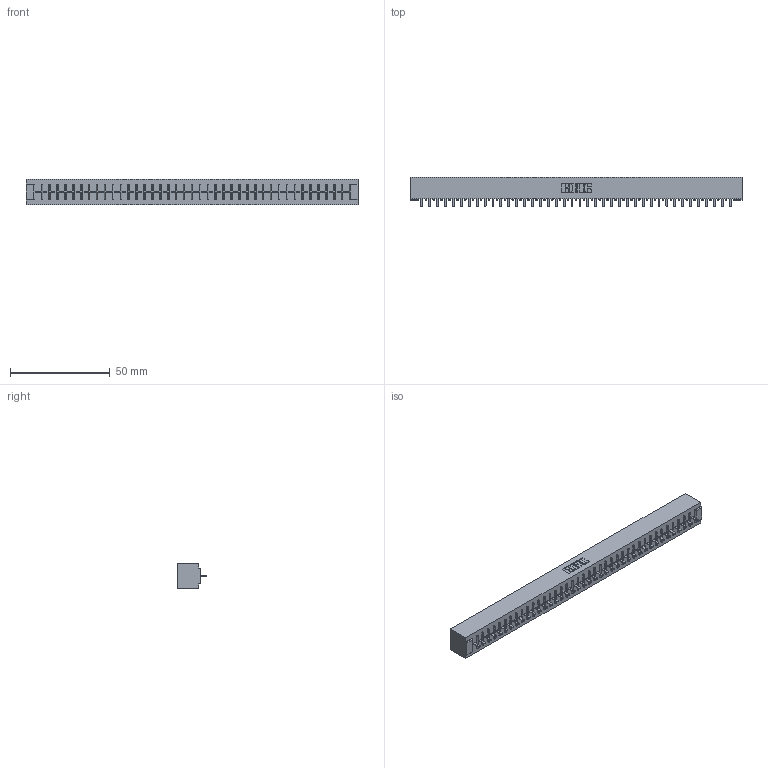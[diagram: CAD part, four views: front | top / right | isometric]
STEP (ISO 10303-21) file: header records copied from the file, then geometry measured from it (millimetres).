
FILE_DESCRIPTION (( 'STEP AP203' ), '1' );
FILE_NAME ('306-040-521-101.STEP', '2019-09-12T00:26:03', ( '' ), ( '' ), 'SwSTEP 2.0', 'SolidWorks 2016', '' );
FILE_SCHEMA (( 'CONFIG_CONTROL_DESIGN' ));
Length unit declared in the file: inch
Products named in the file (3): 306 Part_No Mounting; 306-290-001_121; 306-040-521-101
Assembly tree (41 placements, depth 2):
  306-040-521-101
    306 Part_No Mounting
    306-290-001_121  x40
Bounding box: 166.37 x 14.88 x 12.7 mm (x, y, z)
Volume: 18908.3 mm3; surface area: 19238.3 mm2
Topology: 41 solids, 41 shells, 2908 faces, 8172 edges, 5232 vertices
Faces by surface type: plane 1944, cylinder 804, sphere 160
Entity records: 37239 total; most frequent: CARTESIAN_POINT 6251, ORIENTED_EDGE 6196, DIRECTION 6164, EDGE_CURVE 3098, VECTOR 2426, LINE 2426, VERTEX_POINT 1956, AXIS2_PLACEMENT_3D 1869
